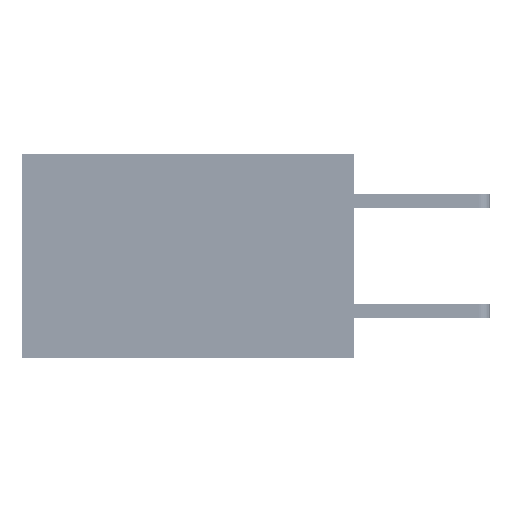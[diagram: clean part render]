
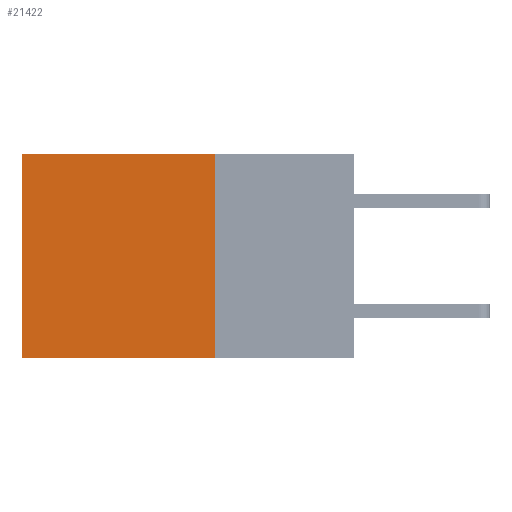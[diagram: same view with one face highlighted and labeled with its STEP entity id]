
A CAD part, left-side view. The second image highlights one B-rep face of the part: STEP entity #21422.
In plain terms, the highlighted planar face has unit normal (-1, 0, 0).
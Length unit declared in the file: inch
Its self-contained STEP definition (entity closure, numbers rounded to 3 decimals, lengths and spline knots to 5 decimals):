
#1716 = VERTEX_POINT ( 'NONE', #34768 ) ;
#2284 = DIRECTION ( 'NONE',  ( 0., 1., 0. ) ) ;
#2788 = DIRECTION ( 'NONE',  ( 1., 0., 0. ) ) ;
#5033 = VERTEX_POINT ( 'NONE', #40159 ) ;
#7898 = CARTESIAN_POINT ( 'NONE',  ( 0.2875, 0.6, 0. ) ) ;
#12226 = LINE ( 'NONE', #7898, #24416 ) ;
#13194 = LINE ( 'NONE', #20490, #31193 ) ;
#13267 = CARTESIAN_POINT ( 'NONE',  ( 0.2875, 0.25, 0. ) ) ;
#14121 = VECTOR ( 'NONE', #35759, 39.37008 ) ;
#14995 = LINE ( 'NONE', #21853, #14121 ) ;
#15533 = ORIENTED_EDGE ( 'NONE', *, *, #44737, .F. ) ;
#20490 = CARTESIAN_POINT ( 'NONE',  ( 0.2875, 0.25, 0. ) ) ;
#21372 = VERTEX_POINT ( 'NONE', #28585 ) ;
#21422 = ADVANCED_FACE ( 'NONE', ( #33355 ), #43847, .F. ) ;
#21801 = DIRECTION ( 'NONE',  ( 0., 0., -1. ) ) ;
#21853 = CARTESIAN_POINT ( 'NONE',  ( 0.2875, 0.25, -0.37 ) ) ;
#22451 = EDGE_LOOP ( 'NONE', ( #32345, #33770, #15533, #23596 ) ) ;
#22775 = VERTEX_POINT ( 'NONE', #43682 ) ;
#23596 = ORIENTED_EDGE ( 'NONE', *, *, #25441, .T. ) ;
#24416 = VECTOR ( 'NONE', #21801, 39.37008 ) ;
#25441 = EDGE_CURVE ( 'NONE', #22775, #1716, #13194, .T. ) ;
#25459 = VECTOR ( 'NONE', #40914, 39.37008 ) ;
#28152 = AXIS2_PLACEMENT_3D ( 'NONE', #13267, #2788, #43625 ) ;
#28585 = CARTESIAN_POINT ( 'NONE',  ( 0.2875, 0.6, -0.37 ) ) ;
#31193 = VECTOR ( 'NONE', #2284, 39.37008 ) ;
#32345 = ORIENTED_EDGE ( 'NONE', *, *, #38128, .T. ) ;
#33173 = CARTESIAN_POINT ( 'NONE',  ( 0.2875, 0.25, 0. ) ) ;
#33355 = FACE_OUTER_BOUND ( 'NONE', #22451, .T. ) ;
#33770 = ORIENTED_EDGE ( 'NONE', *, *, #36941, .F. ) ;
#34768 = CARTESIAN_POINT ( 'NONE',  ( 0.2875, 0.6, 0. ) ) ;
#35759 = DIRECTION ( 'NONE',  ( 0., 1., 0. ) ) ;
#36941 = EDGE_CURVE ( 'NONE', #5033, #21372, #14995, .T. ) ;
#37501 = LINE ( 'NONE', #33173, #25459 ) ;
#38128 = EDGE_CURVE ( 'NONE', #1716, #21372, #12226, .T. ) ;
#40159 = CARTESIAN_POINT ( 'NONE',  ( 0.2875, 0.25, -0.37 ) ) ;
#40914 = DIRECTION ( 'NONE',  ( 0., 0., -1. ) ) ;
#43625 = DIRECTION ( 'NONE',  ( 0., 0., -1. ) ) ;
#43682 = CARTESIAN_POINT ( 'NONE',  ( 0.2875, 0.25, 0. ) ) ;
#43847 = PLANE ( 'NONE',  #28152 ) ;
#44737 = EDGE_CURVE ( 'NONE', #22775, #5033, #37501, .T. ) ;
